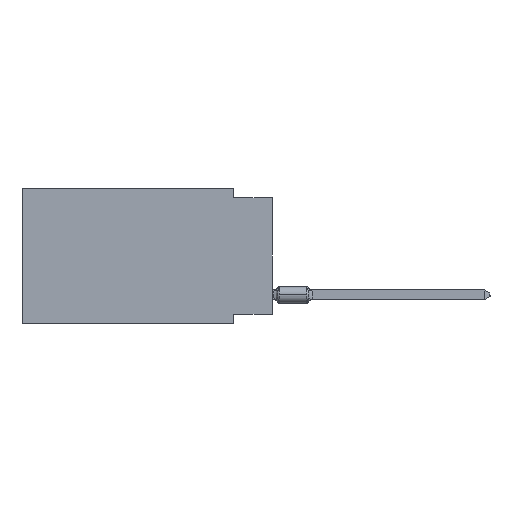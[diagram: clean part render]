
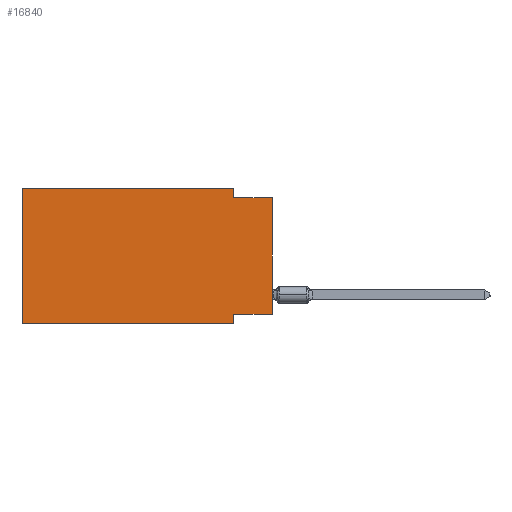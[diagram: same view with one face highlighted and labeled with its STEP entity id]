
A CAD part, left-side view. The second image highlights one B-rep face of the part: STEP entity #16840.
In plain terms, the highlighted planar face has unit normal (-1, 0, 0).
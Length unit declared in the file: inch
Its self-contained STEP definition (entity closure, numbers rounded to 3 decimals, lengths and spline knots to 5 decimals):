
#163 = EDGE_CURVE ( 'NONE', #26546, #8906, #6865, .T. ) ;
#1679 = EDGE_CURVE ( 'NONE', #34461, #4220, #30336, .T. ) ;
#1801 = VERTEX_POINT ( 'NONE', #31776 ) ;
#2050 = ORIENTED_EDGE ( 'NONE', *, *, #163, .T. ) ;
#2555 = EDGE_CURVE ( 'NONE', #1801, #26868, #34545, .T. ) ;
#2695 = ORIENTED_EDGE ( 'NONE', *, *, #14059, .F. ) ;
#4220 = VERTEX_POINT ( 'NONE', #34490 ) ;
#4919 = DIRECTION ( 'NONE',  ( 0., 0., -1. ) ) ;
#5039 = DIRECTION ( 'NONE',  ( 0., -1., 0. ) ) ;
#5522 = VERTEX_POINT ( 'NONE', #22850 ) ;
#5987 = LINE ( 'NONE', #28621, #15478 ) ;
#6865 = LINE ( 'NONE', #35977, #7107 ) ;
#7107 = VECTOR ( 'NONE', #18903, 39.37008 ) ;
#7447 = ORIENTED_EDGE ( 'NONE', *, *, #31223, .F. ) ;
#7704 = PLANE ( 'NONE',  #21579 ) ;
#7893 = FACE_OUTER_BOUND ( 'NONE', #22764, .T. ) ;
#8438 = CARTESIAN_POINT ( 'NONE',  ( 0., 0., -0.025 ) ) ;
#8906 = VERTEX_POINT ( 'NONE', #12458 ) ;
#9119 = CARTESIAN_POINT ( 'NONE',  ( 0., 0.1, -0.025 ) ) ;
#9135 = DIRECTION ( 'NONE',  ( 0., 0., -1. ) ) ;
#9606 = VECTOR ( 'NONE', #4919, 39.37008 ) ;
#10207 = CARTESIAN_POINT ( 'NONE',  ( 0., 0.645, -0.35 ) ) ;
#10311 = DIRECTION ( 'NONE',  ( 1., 0., 0. ) ) ;
#10399 = DIRECTION ( 'NONE',  ( 0., -1., 0. ) ) ;
#10667 = CARTESIAN_POINT ( 'NONE',  ( 0., 0.645, 0. ) ) ;
#11035 = DIRECTION ( 'NONE',  ( 0., -1., 0. ) ) ;
#12075 = DIRECTION ( 'NONE',  ( 0., 0., 1. ) ) ;
#12458 = CARTESIAN_POINT ( 'NONE',  ( 0., 0., -0.025 ) ) ;
#12683 = CARTESIAN_POINT ( 'NONE',  ( 0., 0., -0.325 ) ) ;
#14059 = EDGE_CURVE ( 'NONE', #26868, #8906, #30705, .T. ) ;
#14156 = ORIENTED_EDGE ( 'NONE', *, *, #16460, .T. ) ;
#15198 = CARTESIAN_POINT ( 'NONE',  ( 0., 0.645, -0.35 ) ) ;
#15478 = VECTOR ( 'NONE', #12075, 39.37008 ) ;
#16460 = EDGE_CURVE ( 'NONE', #28574, #4220, #35811, .T. ) ;
#16840 = ADVANCED_FACE ( 'NONE', ( #7893 ), #7704, .F. ) ;
#17651 = CARTESIAN_POINT ( 'NONE',  ( 0., 0.1, 0. ) ) ;
#18540 = ORIENTED_EDGE ( 'NONE', *, *, #22017, .F. ) ;
#18759 = LINE ( 'NONE', #30628, #24912 ) ;
#18903 = DIRECTION ( 'NONE',  ( 0., 0., 1. ) ) ;
#20755 = ORIENTED_EDGE ( 'NONE', *, *, #2555, .F. ) ;
#21579 = AXIS2_PLACEMENT_3D ( 'NONE', #10667, #10311, #25139 ) ;
#22017 = EDGE_CURVE ( 'NONE', #26546, #34461, #23625, .T. ) ;
#22764 = EDGE_LOOP ( 'NONE', ( #2050, #2695, #20755, #24337, #7447, #14156, #28363, #18540 ) ) ;
#22850 = CARTESIAN_POINT ( 'NONE',  ( 0., 0.645, 0. ) ) ;
#23625 = LINE ( 'NONE', #12683, #27224 ) ;
#24007 = DIRECTION ( 'NONE',  ( 0., 1., 0. ) ) ;
#24042 = CARTESIAN_POINT ( 'NONE',  ( 0., 0.1, -0.325 ) ) ;
#24178 = CARTESIAN_POINT ( 'NONE',  ( 0., 0., -0.325 ) ) ;
#24337 = ORIENTED_EDGE ( 'NONE', *, *, #30241, .F. ) ;
#24912 = VECTOR ( 'NONE', #5039, 39.37008 ) ;
#25139 = DIRECTION ( 'NONE',  ( 0., 0., -1. ) ) ;
#26546 = VERTEX_POINT ( 'NONE', #24178 ) ;
#26868 = VERTEX_POINT ( 'NONE', #9119 ) ;
#26912 = VECTOR ( 'NONE', #10399, 39.37008 ) ;
#27224 = VECTOR ( 'NONE', #24007, 39.37008 ) ;
#28052 = VECTOR ( 'NONE', #9135, 39.37008 ) ;
#28363 = ORIENTED_EDGE ( 'NONE', *, *, #1679, .F. ) ;
#28574 = VERTEX_POINT ( 'NONE', #15198 ) ;
#28621 = CARTESIAN_POINT ( 'NONE',  ( 0., 0.645, 0. ) ) ;
#30241 = EDGE_CURVE ( 'NONE', #5522, #1801, #18759, .T. ) ;
#30336 = LINE ( 'NONE', #36263, #9606 ) ;
#30628 = CARTESIAN_POINT ( 'NONE',  ( 0., 0.645, 0. ) ) ;
#30705 = LINE ( 'NONE', #8438, #35834 ) ;
#31223 = EDGE_CURVE ( 'NONE', #28574, #5522, #5987, .T. ) ;
#31776 = CARTESIAN_POINT ( 'NONE',  ( 0., 0.1, 0. ) ) ;
#34461 = VERTEX_POINT ( 'NONE', #24042 ) ;
#34490 = CARTESIAN_POINT ( 'NONE',  ( 0., 0.1, -0.35 ) ) ;
#34545 = LINE ( 'NONE', #17651, #28052 ) ;
#35811 = LINE ( 'NONE', #10207, #26912 ) ;
#35834 = VECTOR ( 'NONE', #11035, 39.37008 ) ;
#35977 = CARTESIAN_POINT ( 'NONE',  ( 0., 0., 0. ) ) ;
#36263 = CARTESIAN_POINT ( 'NONE',  ( 0., 0.1, -0.35 ) ) ;
